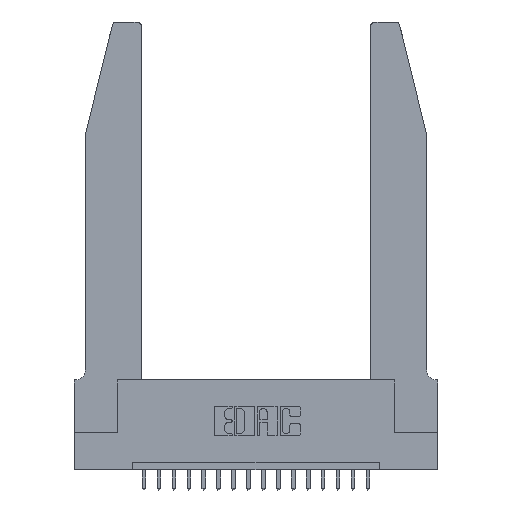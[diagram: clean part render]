
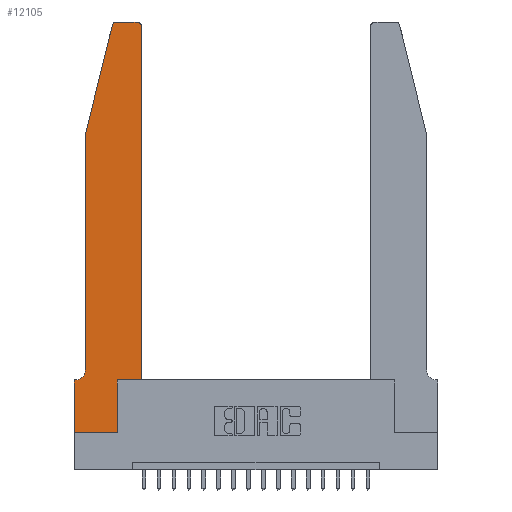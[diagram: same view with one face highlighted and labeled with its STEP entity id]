
A CAD part, top view. The second image highlights one B-rep face of the part: STEP entity #12105.
In plain terms, the highlighted planar face has unit normal (0, 0, 1).
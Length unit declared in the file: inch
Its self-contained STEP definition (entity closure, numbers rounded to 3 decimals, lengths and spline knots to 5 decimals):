
#262 = AXIS2_PLACEMENT_3D ( 'NONE', #20192, #3167, #13967 ) ;
#982 = VERTEX_POINT ( 'NONE', #10659 ) ;
#1266 = LINE ( 'NONE', #13979, #17452 ) ;
#1331 = VECTOR ( 'NONE', #10385, 39.37008 ) ;
#1656 = CARTESIAN_POINT ( 'NONE',  ( 0.0055, 0.42, 0.37 ) ) ;
#1816 = VECTOR ( 'NONE', #7138, 39.37008 ) ;
#1872 = DIRECTION ( 'NONE',  ( 0., 0., -1. ) ) ;
#1964 = EDGE_CURVE ( 'NONE', #11742, #17600, #2070, .T. ) ;
#2070 = LINE ( 'NONE', #17974, #1816 ) ;
#2138 = CARTESIAN_POINT ( 'NONE',  ( 0.284, 2.75, 0.37 ) ) ;
#2399 = VECTOR ( 'NONE', #8973, 39.37008 ) ;
#2400 = EDGE_LOOP ( 'NONE', ( #4231, #9529, #11692, #16080, #19902, #2405, #18302, #15093, #4620, #7307, #13592, #12184 ) ) ;
#2405 = ORIENTED_EDGE ( 'NONE', *, *, #16246, .T. ) ;
#2649 = VERTEX_POINT ( 'NONE', #5268 ) ;
#2996 = EDGE_CURVE ( 'NONE', #16946, #11742, #11574, .T. ) ;
#3070 = DIRECTION ( 'NONE',  ( 0., -1., 0. ) ) ;
#3147 = CARTESIAN_POINT ( 'NONE',  ( 0.2865, 0., 0.37 ) ) ;
#3167 = DIRECTION ( 'NONE',  ( 0., 0., 1. ) ) ;
#3268 = VECTOR ( 'NONE', #3070, 39.37008 ) ;
#3345 = CARTESIAN_POINT ( 'NONE',  ( 0., 0., 0.37 ) ) ;
#3474 = VECTOR ( 'NONE', #6782, 39.37008 ) ;
#3649 = DIRECTION ( 'NONE',  ( 1., 0., 0. ) ) ;
#3666 = AXIS2_PLACEMENT_3D ( 'NONE', #8441, #16436, #3649 ) ;
#3753 = EDGE_CURVE ( 'NONE', #16144, #2649, #19634, .T. ) ;
#3908 = CARTESIAN_POINT ( 'NONE',  ( 0.0755, 2., 0.37 ) ) ;
#4231 = ORIENTED_EDGE ( 'NONE', *, *, #14702, .T. ) ;
#4388 = CARTESIAN_POINT ( 'NONE',  ( 0.0755, 0.42, 0.37 ) ) ;
#4542 = DIRECTION ( 'NONE',  ( 0., 1., 0. ) ) ;
#4620 = ORIENTED_EDGE ( 'NONE', *, *, #20009, .T. ) ;
#5268 = CARTESIAN_POINT ( 'NONE',  ( 0.25487, 2.72718, 0.37 ) ) ;
#5791 = VECTOR ( 'NONE', #6015, 39.37008 ) ;
#6015 = DIRECTION ( 'NONE',  ( -0.239, -0.971, 0. ) ) ;
#6030 = VERTEX_POINT ( 'NONE', #13919 ) ;
#6086 = AXIS2_PLACEMENT_3D ( 'NONE', #1656, #1872, #8180 ) ;
#6106 = CARTESIAN_POINT ( 'NONE',  ( 0.4205, 2.75, 0.37 ) ) ;
#6259 = DIRECTION ( 'NONE',  ( -1., 0., 0. ) ) ;
#6782 = DIRECTION ( 'NONE',  ( 1., 0., 0. ) ) ;
#7045 = EDGE_CURVE ( 'NONE', #982, #7609, #16446, .T. ) ;
#7138 = DIRECTION ( 'NONE',  ( 1., 0., 0. ) ) ;
#7281 = EDGE_CURVE ( 'NONE', #6030, #19843, #13240, .T. ) ;
#7307 = ORIENTED_EDGE ( 'NONE', *, *, #7045, .T. ) ;
#7609 = VERTEX_POINT ( 'NONE', #16899 ) ;
#7846 = CARTESIAN_POINT ( 'NONE',  ( 0.4505, 0.35, 0.37 ) ) ;
#8096 = DIRECTION ( 'NONE',  ( 0., 1., 0. ) ) ;
#8099 = EDGE_CURVE ( 'NONE', #7609, #6030, #8603, .T. ) ;
#8180 = DIRECTION ( 'NONE',  ( -1., 0., 0. ) ) ;
#8441 = CARTESIAN_POINT ( 'NONE',  ( 0.284, 2.72, 0.37 ) ) ;
#8449 = CARTESIAN_POINT ( 'NONE',  ( 0., 0.35, 0.37 ) ) ;
#8534 = CARTESIAN_POINT ( 'NONE',  ( 0.4505, 0.35, 0.37 ) ) ;
#8603 = LINE ( 'NONE', #7846, #15469 ) ;
#8973 = DIRECTION ( 'NONE',  ( 0., -1., 0. ) ) ;
#9513 = EDGE_CURVE ( 'NONE', #16049, #18665, #17341, .T. ) ;
#9529 = ORIENTED_EDGE ( 'NONE', *, *, #3753, .T. ) ;
#10249 = CARTESIAN_POINT ( 'NONE',  ( 0.4205, 2.72, 0.37 ) ) ;
#10354 = CARTESIAN_POINT ( 'NONE',  ( 0.0055, 0.35, 0.37 ) ) ;
#10385 = DIRECTION ( 'NONE',  ( -1., 0., 0. ) ) ;
#10453 = CARTESIAN_POINT ( 'NONE',  ( 0.0755, 2., 0.37 ) ) ;
#10659 = CARTESIAN_POINT ( 'NONE',  ( 0.2865, 0.35, 0.37 ) ) ;
#10854 = AXIS2_PLACEMENT_3D ( 'NONE', #10249, #16617, #18250 ) ;
#11084 = PLANE ( 'NONE',  #262 ) ;
#11574 = LINE ( 'NONE', #3345, #3268 ) ;
#11692 = ORIENTED_EDGE ( 'NONE', *, *, #13744, .T. ) ;
#11742 = VERTEX_POINT ( 'NONE', #11858 ) ;
#11858 = CARTESIAN_POINT ( 'NONE',  ( 0., 0., 0.37 ) ) ;
#11971 = CARTESIAN_POINT ( 'NONE',  ( 0.0755, 2., 0.37 ) ) ;
#12105 = ADVANCED_FACE ( 'NONE', ( #15869 ), #11084, .T. ) ;
#12184 = ORIENTED_EDGE ( 'NONE', *, *, #7281, .T. ) ;
#13240 = CIRCLE ( 'NONE', #10854, 0.03 ) ;
#13435 = LINE ( 'NONE', #19105, #19799 ) ;
#13592 = ORIENTED_EDGE ( 'NONE', *, *, #8099, .T. ) ;
#13616 = LINE ( 'NONE', #3908, #5791 ) ;
#13744 = EDGE_CURVE ( 'NONE', #2649, #16049, #13616, .T. ) ;
#13817 = CIRCLE ( 'NONE', #6086, 0.07 ) ;
#13822 = CARTESIAN_POINT ( 'NONE',  ( 0.2605, 2.75, 0.37 ) ) ;
#13919 = CARTESIAN_POINT ( 'NONE',  ( 0.4505, 2.72, 0.37 ) ) ;
#13967 = DIRECTION ( 'NONE',  ( 1., 0., 0. ) ) ;
#13979 = CARTESIAN_POINT ( 'NONE',  ( 0.0755, 0.35, 0.37 ) ) ;
#14139 = VERTEX_POINT ( 'NONE', #10354 ) ;
#14702 = EDGE_CURVE ( 'NONE', #19843, #16144, #16289, .T. ) ;
#14976 = EDGE_CURVE ( 'NONE', #18665, #14139, #13817, .T. ) ;
#15093 = ORIENTED_EDGE ( 'NONE', *, *, #1964, .T. ) ;
#15469 = VECTOR ( 'NONE', #4542, 39.37008 ) ;
#15869 = FACE_OUTER_BOUND ( 'NONE', #2400, .T. ) ;
#16049 = VERTEX_POINT ( 'NONE', #11971 ) ;
#16080 = ORIENTED_EDGE ( 'NONE', *, *, #9513, .T. ) ;
#16144 = VERTEX_POINT ( 'NONE', #2138 ) ;
#16246 = EDGE_CURVE ( 'NONE', #14139, #16946, #1266, .T. ) ;
#16289 = LINE ( 'NONE', #13822, #1331 ) ;
#16436 = DIRECTION ( 'NONE',  ( 0., 0., 1. ) ) ;
#16446 = LINE ( 'NONE', #8534, #3474 ) ;
#16617 = DIRECTION ( 'NONE',  ( 0., 0., 1. ) ) ;
#16899 = CARTESIAN_POINT ( 'NONE',  ( 0.4505, 0.35, 0.37 ) ) ;
#16946 = VERTEX_POINT ( 'NONE', #8449 ) ;
#17341 = LINE ( 'NONE', #10453, #2399 ) ;
#17452 = VECTOR ( 'NONE', #6259, 39.37008 ) ;
#17600 = VERTEX_POINT ( 'NONE', #3147 ) ;
#17974 = CARTESIAN_POINT ( 'NONE',  ( 0., 0., 0.37 ) ) ;
#18250 = DIRECTION ( 'NONE',  ( 1., 0., 0. ) ) ;
#18302 = ORIENTED_EDGE ( 'NONE', *, *, #2996, .T. ) ;
#18665 = VERTEX_POINT ( 'NONE', #4388 ) ;
#19105 = CARTESIAN_POINT ( 'NONE',  ( 0.2865, 0.35, 0.37 ) ) ;
#19634 = CIRCLE ( 'NONE', #3666, 0.03 ) ;
#19799 = VECTOR ( 'NONE', #8096, 39.37008 ) ;
#19843 = VERTEX_POINT ( 'NONE', #6106 ) ;
#19902 = ORIENTED_EDGE ( 'NONE', *, *, #14976, .T. ) ;
#20009 = EDGE_CURVE ( 'NONE', #17600, #982, #13435, .T. ) ;
#20192 = CARTESIAN_POINT ( 'NONE',  ( 0., 0.35, 0.37 ) ) ;
